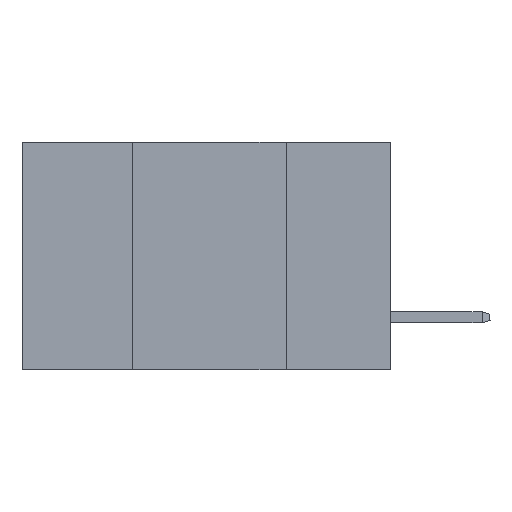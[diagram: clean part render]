
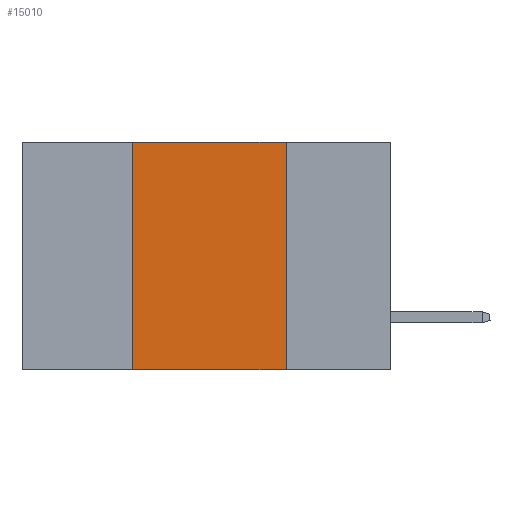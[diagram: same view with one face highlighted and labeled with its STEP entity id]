
A CAD part, left-side view. The second image highlights one B-rep face of the part: STEP entity #15010.
In plain terms, the highlighted planar face has unit normal (-1, 0, 0).
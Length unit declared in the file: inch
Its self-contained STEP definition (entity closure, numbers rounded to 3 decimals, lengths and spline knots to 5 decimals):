
#131 = DIRECTION ( 'NONE',  ( 0., 0., -1. ) ) ;
#438 = EDGE_CURVE ( 'NONE', #9900, #18040, #16347, .T. ) ;
#522 = DIRECTION ( 'NONE',  ( 1., 0., 0. ) ) ;
#674 = CARTESIAN_POINT ( 'NONE',  ( 0., 0.6, 0. ) ) ;
#1283 = CARTESIAN_POINT ( 'NONE',  ( 0., 0.42, 0. ) ) ;
#3503 = FACE_OUTER_BOUND ( 'NONE', #19348, .T. ) ;
#3513 = CARTESIAN_POINT ( 'NONE',  ( 0., 0.6, 0. ) ) ;
#4972 = EDGE_CURVE ( 'NONE', #10539, #8621, #15926, .T. ) ;
#5159 = ORIENTED_EDGE ( 'NONE', *, *, #19015, .F. ) ;
#5388 = VECTOR ( 'NONE', #6440, 39.37008 ) ;
#6272 = CARTESIAN_POINT ( 'NONE',  ( 0., 0.17, 0. ) ) ;
#6440 = DIRECTION ( 'NONE',  ( 0., -1., 0. ) ) ;
#6542 = PLANE ( 'NONE',  #16685 ) ;
#8621 = VERTEX_POINT ( 'NONE', #17806 ) ;
#8833 = ORIENTED_EDGE ( 'NONE', *, *, #438, .T. ) ;
#8999 = VECTOR ( 'NONE', #14774, 39.37008 ) ;
#9259 = EDGE_CURVE ( 'NONE', #8621, #18040, #12064, .T. ) ;
#9614 = CARTESIAN_POINT ( 'NONE',  ( 0., 0.42, 0. ) ) ;
#9900 = VERTEX_POINT ( 'NONE', #12376 ) ;
#10539 = VERTEX_POINT ( 'NONE', #9614 ) ;
#10569 = DIRECTION ( 'NONE',  ( 0., -1., 0. ) ) ;
#12035 = ORIENTED_EDGE ( 'NONE', *, *, #4972, .F. ) ;
#12064 = LINE ( 'NONE', #6272, #16032 ) ;
#12354 = VECTOR ( 'NONE', #10569, 39.37008 ) ;
#12376 = CARTESIAN_POINT ( 'NONE',  ( 0., 0.42, -0.37 ) ) ;
#12593 = DIRECTION ( 'NONE',  ( 0., 0., -1. ) ) ;
#14774 = DIRECTION ( 'NONE',  ( 0., 0., 1. ) ) ;
#15010 = ADVANCED_FACE ( 'NONE', ( #3503 ), #6542, .F. ) ;
#15169 = ORIENTED_EDGE ( 'NONE', *, *, #9259, .F. ) ;
#15275 = CARTESIAN_POINT ( 'NONE',  ( 0., 0.6, -0.37 ) ) ;
#15926 = LINE ( 'NONE', #3513, #5388 ) ;
#16032 = VECTOR ( 'NONE', #131, 39.37008 ) ;
#16347 = LINE ( 'NONE', #15275, #12354 ) ;
#16685 = AXIS2_PLACEMENT_3D ( 'NONE', #674, #522, #12593 ) ;
#16954 = LINE ( 'NONE', #1283, #8999 ) ;
#17573 = CARTESIAN_POINT ( 'NONE',  ( 0., 0.17, -0.37 ) ) ;
#17806 = CARTESIAN_POINT ( 'NONE',  ( 0., 0.17, 0. ) ) ;
#18040 = VERTEX_POINT ( 'NONE', #17573 ) ;
#19015 = EDGE_CURVE ( 'NONE', #9900, #10539, #16954, .T. ) ;
#19348 = EDGE_LOOP ( 'NONE', ( #15169, #12035, #5159, #8833 ) ) ;
